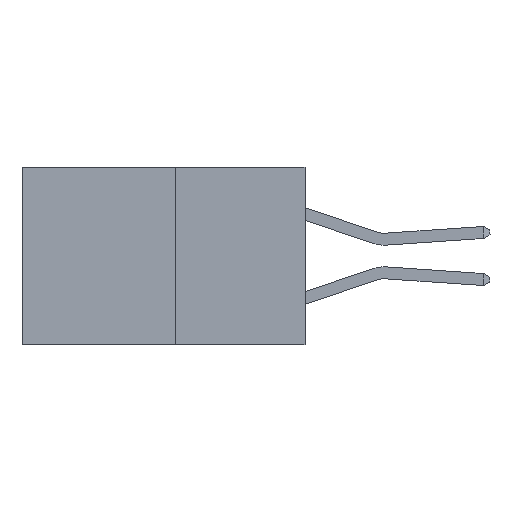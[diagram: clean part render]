
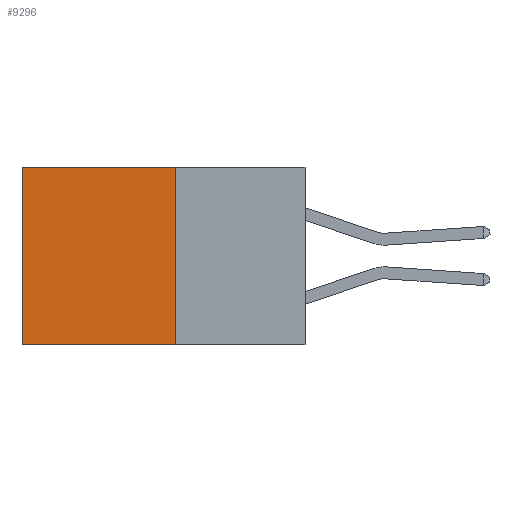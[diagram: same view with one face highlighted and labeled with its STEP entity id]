
A CAD part, left-side view. The second image highlights one B-rep face of the part: STEP entity #9296.
In plain terms, the highlighted planar face has unit normal (-1, 0, 0).
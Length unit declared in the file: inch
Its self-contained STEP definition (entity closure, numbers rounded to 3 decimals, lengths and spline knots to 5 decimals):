
#289 = ORIENTED_EDGE ( 'NONE', *, *, #14950, .F. ) ;
#1824 = CARTESIAN_POINT ( 'NONE',  ( 0.277, 0.27, 0. ) ) ;
#2077 = DIRECTION ( 'NONE',  ( 0., 1., 0. ) ) ;
#2620 = VECTOR ( 'NONE', #5924, 39.37008 ) ;
#3815 = DIRECTION ( 'NONE',  ( 0., 0., -1. ) ) ;
#5291 = VECTOR ( 'NONE', #2077, 39.37008 ) ;
#5924 = DIRECTION ( 'NONE',  ( 0., 0., -1. ) ) ;
#6386 = LINE ( 'NONE', #14150, #5291 ) ;
#6504 = VERTEX_POINT ( 'NONE', #18015 ) ;
#7419 = VECTOR ( 'NONE', #3815, 39.37008 ) ;
#7564 = VECTOR ( 'NONE', #8824, 39.37008 ) ;
#8544 = CARTESIAN_POINT ( 'NONE',  ( 0.277, 0.27, -0.37 ) ) ;
#8824 = DIRECTION ( 'NONE',  ( 0., 1., 0. ) ) ;
#9296 = ADVANCED_FACE ( 'NONE', ( #10682 ), #21868, .F. ) ;
#10211 = DIRECTION ( 'NONE',  ( 0., 0., -1. ) ) ;
#10682 = FACE_OUTER_BOUND ( 'NONE', #14685, .T. ) ;
#11329 = VERTEX_POINT ( 'NONE', #19089 ) ;
#12330 = CARTESIAN_POINT ( 'NONE',  ( 0.277, 0.27, -0.37 ) ) ;
#12487 = LINE ( 'NONE', #12330, #7419 ) ;
#12576 = EDGE_CURVE ( 'NONE', #20145, #15600, #6386, .T. ) ;
#12829 = CARTESIAN_POINT ( 'NONE',  ( 0.277, 0.59, -0.37 ) ) ;
#13347 = AXIS2_PLACEMENT_3D ( 'NONE', #8544, #20292, #10211 ) ;
#13798 = CARTESIAN_POINT ( 'NONE',  ( 0.277, 0.59, -0.37 ) ) ;
#14150 = CARTESIAN_POINT ( 'NONE',  ( 0.277, 0.27, -0.37 ) ) ;
#14685 = EDGE_LOOP ( 'NONE', ( #19542, #16497, #289, #15593 ) ) ;
#14950 = EDGE_CURVE ( 'NONE', #11329, #20145, #12487, .T. ) ;
#15034 = CARTESIAN_POINT ( 'NONE',  ( 0.277, 0.27, -0.37 ) ) ;
#15593 = ORIENTED_EDGE ( 'NONE', *, *, #19694, .T. ) ;
#15600 = VERTEX_POINT ( 'NONE', #13798 ) ;
#16497 = ORIENTED_EDGE ( 'NONE', *, *, #12576, .F. ) ;
#16580 = LINE ( 'NONE', #1824, #7564 ) ;
#18015 = CARTESIAN_POINT ( 'NONE',  ( 0.277, 0.59, 0. ) ) ;
#19089 = CARTESIAN_POINT ( 'NONE',  ( 0.277, 0.27, 0. ) ) ;
#19542 = ORIENTED_EDGE ( 'NONE', *, *, #19956, .T. ) ;
#19694 = EDGE_CURVE ( 'NONE', #11329, #6504, #16580, .T. ) ;
#19956 = EDGE_CURVE ( 'NONE', #6504, #15600, #20707, .T. ) ;
#20145 = VERTEX_POINT ( 'NONE', #15034 ) ;
#20292 = DIRECTION ( 'NONE',  ( 1., 0., 0. ) ) ;
#20707 = LINE ( 'NONE', #12829, #2620 ) ;
#21868 = PLANE ( 'NONE',  #13347 ) ;
